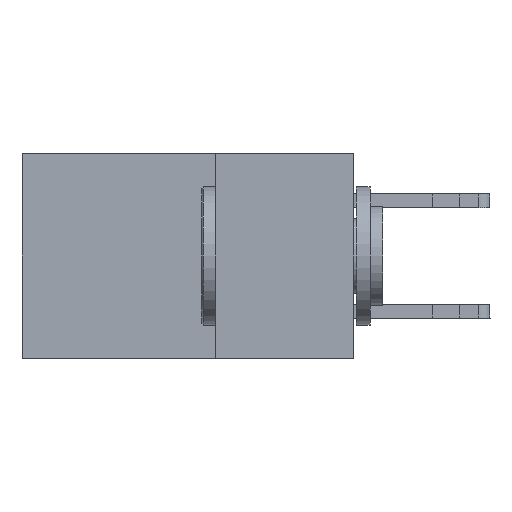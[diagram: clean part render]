
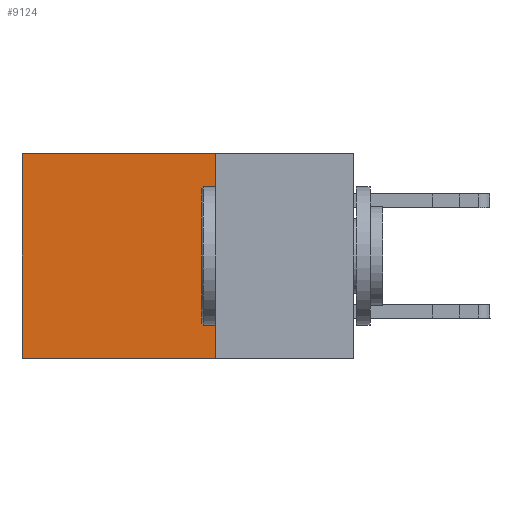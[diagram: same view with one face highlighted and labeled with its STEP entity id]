
A CAD part, left-side view. The second image highlights one B-rep face of the part: STEP entity #9124.
In plain terms, the highlighted planar face has unit normal (-1, 0, 0).
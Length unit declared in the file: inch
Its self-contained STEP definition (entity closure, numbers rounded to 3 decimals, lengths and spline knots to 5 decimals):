
#185 = DIRECTION ( 'NONE',  ( 1., 0., 0. ) ) ;
#1021 = FACE_OUTER_BOUND ( 'NONE', #8386, .T. ) ;
#1591 = LINE ( 'NONE', #10228, #12915 ) ;
#1933 = CARTESIAN_POINT ( 'NONE',  ( 0.2875, 0.25, 0. ) ) ;
#2055 = CARTESIAN_POINT ( 'NONE',  ( 0.2875, 0.25, 0. ) ) ;
#2278 = DIRECTION ( 'NONE',  ( 0., 0., -1. ) ) ;
#3548 = EDGE_CURVE ( 'NONE', #13588, #6081, #1591, .T. ) ;
#4140 = DIRECTION ( 'NONE',  ( 0., 0., -1. ) ) ;
#5147 = VECTOR ( 'NONE', #11419, 39.37008 ) ;
#5538 = CARTESIAN_POINT ( 'NONE',  ( 0.2875, 0.25, -0.37 ) ) ;
#6002 = EDGE_CURVE ( 'NONE', #14560, #6081, #6187, .T. ) ;
#6081 = VERTEX_POINT ( 'NONE', #16498 ) ;
#6187 = LINE ( 'NONE', #5538, #9112 ) ;
#6708 = ORIENTED_EDGE ( 'NONE', *, *, #3548, .T. ) ;
#8126 = DIRECTION ( 'NONE',  ( 0., 0., -1. ) ) ;
#8134 = PLANE ( 'NONE',  #9327 ) ;
#8386 = EDGE_LOOP ( 'NONE', ( #6708, #15288, #10241, #12924 ) ) ;
#8784 = DIRECTION ( 'NONE',  ( 0., 1., 0. ) ) ;
#9112 = VECTOR ( 'NONE', #8784, 39.37008 ) ;
#9124 = ADVANCED_FACE ( 'NONE', ( #1021 ), #8134, .F. ) ;
#9327 = AXIS2_PLACEMENT_3D ( 'NONE', #12181, #185, #4140 ) ;
#9448 = LINE ( 'NONE', #9588, #10304 ) ;
#9588 = CARTESIAN_POINT ( 'NONE',  ( 0.2875, 0.25, 0. ) ) ;
#10228 = CARTESIAN_POINT ( 'NONE',  ( 0.2875, 0.6, 0. ) ) ;
#10241 = ORIENTED_EDGE ( 'NONE', *, *, #15446, .F. ) ;
#10304 = VECTOR ( 'NONE', #8126, 39.37008 ) ;
#10882 = CARTESIAN_POINT ( 'NONE',  ( 0.2875, 0.25, -0.37 ) ) ;
#10907 = EDGE_CURVE ( 'NONE', #12129, #13588, #13323, .T. ) ;
#11419 = DIRECTION ( 'NONE',  ( 0., 1., 0. ) ) ;
#11750 = CARTESIAN_POINT ( 'NONE',  ( 0.2875, 0.6, 0. ) ) ;
#12129 = VERTEX_POINT ( 'NONE', #1933 ) ;
#12181 = CARTESIAN_POINT ( 'NONE',  ( 0.2875, 0.25, 0. ) ) ;
#12915 = VECTOR ( 'NONE', #2278, 39.37008 ) ;
#12924 = ORIENTED_EDGE ( 'NONE', *, *, #10907, .T. ) ;
#13323 = LINE ( 'NONE', #2055, #5147 ) ;
#13588 = VERTEX_POINT ( 'NONE', #11750 ) ;
#14560 = VERTEX_POINT ( 'NONE', #10882 ) ;
#15288 = ORIENTED_EDGE ( 'NONE', *, *, #6002, .F. ) ;
#15446 = EDGE_CURVE ( 'NONE', #12129, #14560, #9448, .T. ) ;
#16498 = CARTESIAN_POINT ( 'NONE',  ( 0.2875, 0.6, -0.37 ) ) ;
